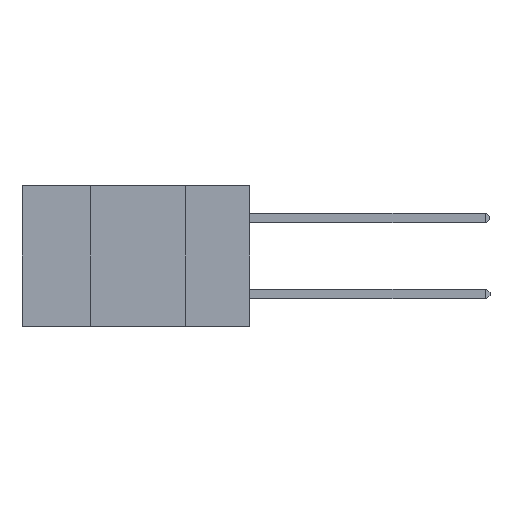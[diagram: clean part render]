
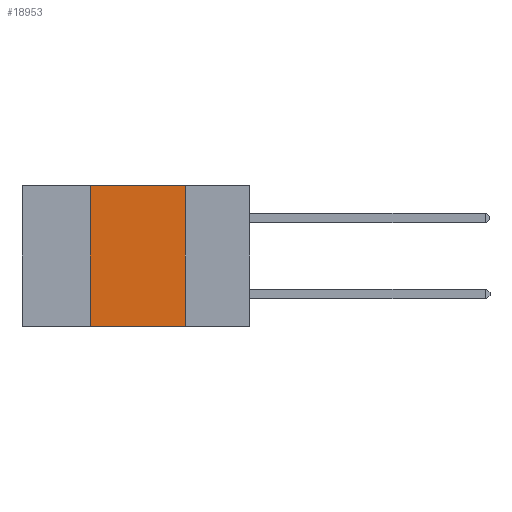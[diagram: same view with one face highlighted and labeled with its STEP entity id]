
A CAD part, left-side view. The second image highlights one B-rep face of the part: STEP entity #18953.
In plain terms, the highlighted planar face has unit normal (-1, 0, 0).
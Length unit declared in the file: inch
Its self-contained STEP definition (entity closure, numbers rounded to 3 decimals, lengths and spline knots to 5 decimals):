
#674 = EDGE_LOOP ( 'NONE', ( #2982, #22517, #18438, #15092 ) ) ;
#1389 = CARTESIAN_POINT ( 'NONE',  ( 0., 0.17, 0. ) ) ;
#1830 = CARTESIAN_POINT ( 'NONE',  ( 0., 0.6, 0. ) ) ;
#2718 = LINE ( 'NONE', #11168, #16514 ) ;
#2982 = ORIENTED_EDGE ( 'NONE', *, *, #5431, .F. ) ;
#4914 = VERTEX_POINT ( 'NONE', #21426 ) ;
#4951 = DIRECTION ( 'NONE',  ( 0., -1., 0. ) ) ;
#5431 = EDGE_CURVE ( 'NONE', #4914, #10837, #20645, .T. ) ;
#5730 = CARTESIAN_POINT ( 'NONE',  ( 0., 0.6, 0. ) ) ;
#5896 = VERTEX_POINT ( 'NONE', #11566 ) ;
#5966 = CARTESIAN_POINT ( 'NONE',  ( 0., 0.17, -0.37 ) ) ;
#7154 = DIRECTION ( 'NONE',  ( 0., -1., 0. ) ) ;
#8925 = VECTOR ( 'NONE', #7154, 39.37008 ) ;
#9292 = DIRECTION ( 'NONE',  ( 0., 0., -1. ) ) ;
#10837 = VERTEX_POINT ( 'NONE', #5966 ) ;
#11168 = CARTESIAN_POINT ( 'NONE',  ( 0., 0.42, 0. ) ) ;
#11566 = CARTESIAN_POINT ( 'NONE',  ( 0., 0.42, -0.37 ) ) ;
#12135 = CARTESIAN_POINT ( 'NONE',  ( 0., 0.42, 0. ) ) ;
#12764 = FACE_OUTER_BOUND ( 'NONE', #674, .T. ) ;
#13165 = VERTEX_POINT ( 'NONE', #12135 ) ;
#14317 = LINE ( 'NONE', #1830, #8925 ) ;
#15092 = ORIENTED_EDGE ( 'NONE', *, *, #20499, .T. ) ;
#16061 = VECTOR ( 'NONE', #4951, 39.37008 ) ;
#16514 = VECTOR ( 'NONE', #21840, 39.37008 ) ;
#17750 = EDGE_CURVE ( 'NONE', #5896, #13165, #2718, .T. ) ;
#17967 = VECTOR ( 'NONE', #19160, 39.37008 ) ;
#18276 = PLANE ( 'NONE',  #20600 ) ;
#18438 = ORIENTED_EDGE ( 'NONE', *, *, #17750, .F. ) ;
#18953 = ADVANCED_FACE ( 'NONE', ( #12764 ), #18276, .F. ) ;
#19160 = DIRECTION ( 'NONE',  ( 0., 0., -1. ) ) ;
#20016 = DIRECTION ( 'NONE',  ( 1., 0., 0. ) ) ;
#20499 = EDGE_CURVE ( 'NONE', #5896, #10837, #20750, .T. ) ;
#20600 = AXIS2_PLACEMENT_3D ( 'NONE', #5730, #20016, #9292 ) ;
#20645 = LINE ( 'NONE', #1389, #17967 ) ;
#20750 = LINE ( 'NONE', #22712, #16061 ) ;
#21426 = CARTESIAN_POINT ( 'NONE',  ( 0., 0.17, 0. ) ) ;
#21840 = DIRECTION ( 'NONE',  ( 0., 0., 1. ) ) ;
#21937 = EDGE_CURVE ( 'NONE', #13165, #4914, #14317, .T. ) ;
#22517 = ORIENTED_EDGE ( 'NONE', *, *, #21937, .F. ) ;
#22712 = CARTESIAN_POINT ( 'NONE',  ( 0., 0.6, -0.37 ) ) ;
